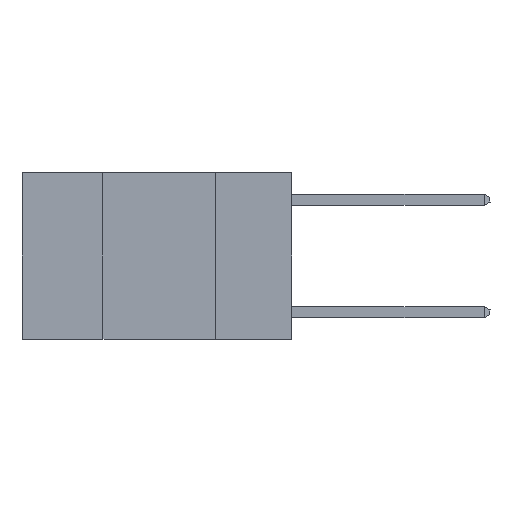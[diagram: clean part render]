
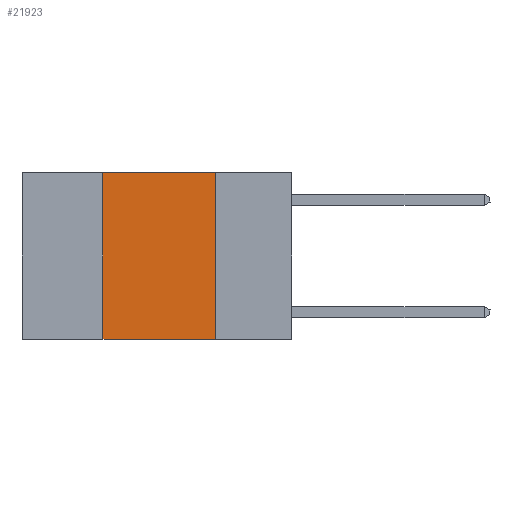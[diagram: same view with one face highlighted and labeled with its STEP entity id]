
A CAD part, left-side view. The second image highlights one B-rep face of the part: STEP entity #21923.
In plain terms, the highlighted planar face has unit normal (-1, 0, 0).
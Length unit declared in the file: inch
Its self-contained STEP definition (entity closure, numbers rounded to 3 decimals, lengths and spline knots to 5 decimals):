
#63 = CARTESIAN_POINT ( 'NONE',  ( 0., 0.42, 0. ) ) ;
#861 = AXIS2_PLACEMENT_3D ( 'NONE', #27168, #5234, #10520 ) ;
#1317 = VECTOR ( 'NONE', #8804, 39.37008 ) ;
#1724 = CARTESIAN_POINT ( 'NONE',  ( 0., 0.17, 0. ) ) ;
#5234 = DIRECTION ( 'NONE',  ( 1., 0., 0. ) ) ;
#6270 = ORIENTED_EDGE ( 'NONE', *, *, #25556, .T. ) ;
#6447 = VERTEX_POINT ( 'NONE', #1724 ) ;
#7254 = EDGE_CURVE ( 'NONE', #6447, #14823, #17958, .T. ) ;
#8804 = DIRECTION ( 'NONE',  ( 0., -1., 0. ) ) ;
#8878 = EDGE_LOOP ( 'NONE', ( #22412, #15213, #26235, #6270 ) ) ;
#9363 = LINE ( 'NONE', #63, #21155 ) ;
#10368 = FACE_OUTER_BOUND ( 'NONE', #8878, .T. ) ;
#10520 = DIRECTION ( 'NONE',  ( 0., 0., -1. ) ) ;
#13858 = CARTESIAN_POINT ( 'NONE',  ( 0., 0.17, -0.37 ) ) ;
#14104 = LINE ( 'NONE', #30748, #1317 ) ;
#14307 = CARTESIAN_POINT ( 'NONE',  ( 0., 0.42, -0.37 ) ) ;
#14823 = VERTEX_POINT ( 'NONE', #13858 ) ;
#15056 = VECTOR ( 'NONE', #31504, 39.37008 ) ;
#15213 = ORIENTED_EDGE ( 'NONE', *, *, #27489, .F. ) ;
#15904 = VECTOR ( 'NONE', #20506, 39.37008 ) ;
#16213 = EDGE_CURVE ( 'NONE', #30260, #31348, #9363, .T. ) ;
#17958 = LINE ( 'NONE', #27704, #15904 ) ;
#20123 = PLANE ( 'NONE',  #861 ) ;
#20506 = DIRECTION ( 'NONE',  ( 0., 0., -1. ) ) ;
#21155 = VECTOR ( 'NONE', #29512, 39.37008 ) ;
#21717 = LINE ( 'NONE', #29390, #15056 ) ;
#21923 = ADVANCED_FACE ( 'NONE', ( #10368 ), #20123, .F. ) ;
#22412 = ORIENTED_EDGE ( 'NONE', *, *, #7254, .F. ) ;
#25556 = EDGE_CURVE ( 'NONE', #30260, #14823, #21717, .T. ) ;
#26235 = ORIENTED_EDGE ( 'NONE', *, *, #16213, .F. ) ;
#27168 = CARTESIAN_POINT ( 'NONE',  ( 0., 0.6, 0. ) ) ;
#27489 = EDGE_CURVE ( 'NONE', #31348, #6447, #14104, .T. ) ;
#27704 = CARTESIAN_POINT ( 'NONE',  ( 0., 0.17, 0. ) ) ;
#27731 = CARTESIAN_POINT ( 'NONE',  ( 0., 0.42, 0. ) ) ;
#29390 = CARTESIAN_POINT ( 'NONE',  ( 0., 0.6, -0.37 ) ) ;
#29512 = DIRECTION ( 'NONE',  ( 0., 0., 1. ) ) ;
#30260 = VERTEX_POINT ( 'NONE', #14307 ) ;
#30748 = CARTESIAN_POINT ( 'NONE',  ( 0., 0.6, 0. ) ) ;
#31348 = VERTEX_POINT ( 'NONE', #27731 ) ;
#31504 = DIRECTION ( 'NONE',  ( 0., -1., 0. ) ) ;
